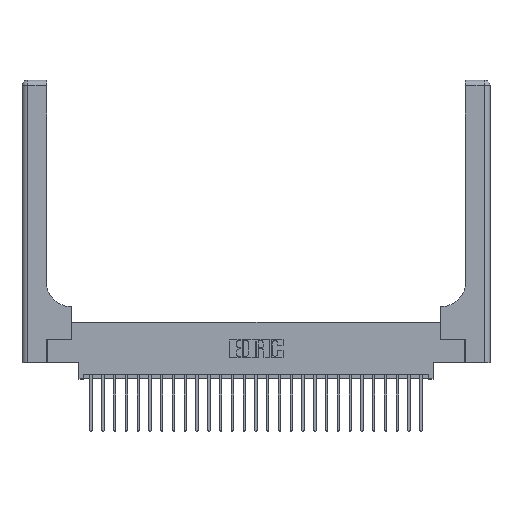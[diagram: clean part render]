
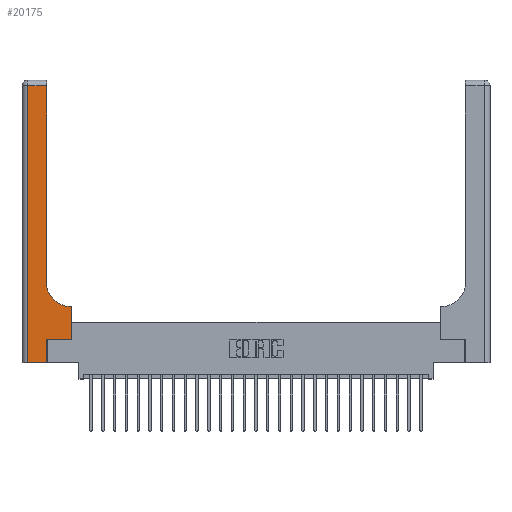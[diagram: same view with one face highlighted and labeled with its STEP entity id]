
A CAD part, top view. The second image highlights one B-rep face of the part: STEP entity #20175.
In plain terms, the highlighted planar face has unit normal (0, 0, 1).
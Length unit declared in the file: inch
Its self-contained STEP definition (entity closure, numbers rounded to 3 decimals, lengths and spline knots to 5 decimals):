
#98 = CARTESIAN_POINT ( 'NONE',  ( 0.528, 0.25, 0.37 ) ) ;
#495 = EDGE_CURVE ( 'NONE', #5238, #13865, #24114, .T. ) ;
#578 = VERTEX_POINT ( 'NONE', #21238 ) ;
#919 = ORIENTED_EDGE ( 'NONE', *, *, #9119, .T. ) ;
#1063 = CARTESIAN_POINT ( 'NONE',  ( 0.265, 0.25, 0.37 ) ) ;
#1071 = DIRECTION ( 'NONE',  ( 1., 0., 0. ) ) ;
#2001 = VERTEX_POINT ( 'NONE', #22235 ) ;
#2119 = VECTOR ( 'NONE', #13141, 39.37008 ) ;
#2160 = VECTOR ( 'NONE', #2380, 39.37008 ) ;
#2380 = DIRECTION ( 'NONE',  ( 0., -1., 0. ) ) ;
#2466 = VERTEX_POINT ( 'NONE', #25644 ) ;
#2586 = EDGE_CURVE ( 'NONE', #578, #5238, #10219, .T. ) ;
#4257 = CARTESIAN_POINT ( 'NONE',  ( 0.26, 2.94, 0.37 ) ) ;
#4840 = LINE ( 'NONE', #10431, #6106 ) ;
#4924 = CARTESIAN_POINT ( 'NONE',  ( 0.265, 0., 0.37 ) ) ;
#5238 = VERTEX_POINT ( 'NONE', #7798 ) ;
#5570 = ORIENTED_EDGE ( 'NONE', *, *, #13798, .T. ) ;
#5649 = ORIENTED_EDGE ( 'NONE', *, *, #495, .T. ) ;
#6106 = VECTOR ( 'NONE', #22444, 39.37008 ) ;
#6125 = ORIENTED_EDGE ( 'NONE', *, *, #25254, .T. ) ;
#7269 = EDGE_LOOP ( 'NONE', ( #13743, #919, #6125, #23512, #5649, #5570, #12803, #18125, #8104 ) ) ;
#7500 = LINE ( 'NONE', #17080, #2119 ) ;
#7531 = VERTEX_POINT ( 'NONE', #12950 ) ;
#7798 = CARTESIAN_POINT ( 'NONE',  ( 0.265, 0., 0.37 ) ) ;
#8031 = DIRECTION ( 'NONE',  ( 0., 0., -1. ) ) ;
#8104 = ORIENTED_EDGE ( 'NONE', *, *, #19860, .T. ) ;
#8174 = LINE ( 'NONE', #14430, #2160 ) ;
#8747 = CARTESIAN_POINT ( 'NONE',  ( 0., 2.94, 0.37 ) ) ;
#8979 = VERTEX_POINT ( 'NONE', #4257 ) ;
#9014 = CARTESIAN_POINT ( 'NONE',  ( 0.265, 0.25, 0.37 ) ) ;
#9119 = EDGE_CURVE ( 'NONE', #8979, #11363, #23045, .T. ) ;
#9296 = VECTOR ( 'NONE', #16214, 39.37008 ) ;
#10219 = LINE ( 'NONE', #13956, #14925 ) ;
#10431 = CARTESIAN_POINT ( 'NONE',  ( 0.26, 3., 0.37 ) ) ;
#10908 = AXIS2_PLACEMENT_3D ( 'NONE', #25143, #13137, #1071 ) ;
#10985 = DIRECTION ( 'NONE',  ( 0., 1., 0. ) ) ;
#11189 = VERTEX_POINT ( 'NONE', #16706 ) ;
#11363 = VERTEX_POINT ( 'NONE', #11869 ) ;
#11869 = CARTESIAN_POINT ( 'NONE',  ( 0.06, 2.94, 0.37 ) ) ;
#11971 = CARTESIAN_POINT ( 'NONE',  ( 0., 3., 0.37 ) ) ;
#12465 = EDGE_CURVE ( 'NONE', #7531, #2466, #7500, .T. ) ;
#12803 = ORIENTED_EDGE ( 'NONE', *, *, #21527, .T. ) ;
#12950 = CARTESIAN_POINT ( 'NONE',  ( 0.528, 0.6, 0.37 ) ) ;
#13097 = AXIS2_PLACEMENT_3D ( 'NONE', #11971, #8031, #22046 ) ;
#13137 = DIRECTION ( 'NONE',  ( 0., 0., -1. ) ) ;
#13141 = DIRECTION ( 'NONE',  ( -1., 0., 0. ) ) ;
#13294 = VECTOR ( 'NONE', #23034, 39.37008 ) ;
#13743 = ORIENTED_EDGE ( 'NONE', *, *, #22716, .T. ) ;
#13798 = EDGE_CURVE ( 'NONE', #13865, #2001, #17975, .T. ) ;
#13865 = VERTEX_POINT ( 'NONE', #1063 ) ;
#13956 = CARTESIAN_POINT ( 'NONE',  ( 0., 0., 0.37 ) ) ;
#14430 = CARTESIAN_POINT ( 'NONE',  ( 0.06, 3., 0.37 ) ) ;
#14925 = VECTOR ( 'NONE', #17988, 39.37008 ) ;
#15609 = FACE_OUTER_BOUND ( 'NONE', #7269, .T. ) ;
#16214 = DIRECTION ( 'NONE',  ( 0., 1., 0. ) ) ;
#16706 = CARTESIAN_POINT ( 'NONE',  ( 0.26, 0.85, 0.37 ) ) ;
#17080 = CARTESIAN_POINT ( 'NONE',  ( 0.26, 0.6, 0.37 ) ) ;
#17975 = LINE ( 'NONE', #9014, #13294 ) ;
#17988 = DIRECTION ( 'NONE',  ( 1., 0., 0. ) ) ;
#18125 = ORIENTED_EDGE ( 'NONE', *, *, #12465, .T. ) ;
#18340 = VECTOR ( 'NONE', #22765, 39.37008 ) ;
#19860 = EDGE_CURVE ( 'NONE', #2466, #11189, #22528, .T. ) ;
#20035 = PLANE ( 'NONE',  #13097 ) ;
#20175 = ADVANCED_FACE ( 'NONE', ( #15609 ), #20035, .F. ) ;
#21238 = CARTESIAN_POINT ( 'NONE',  ( 0.06, 0., 0.37 ) ) ;
#21527 = EDGE_CURVE ( 'NONE', #2001, #7531, #25932, .T. ) ;
#22046 = DIRECTION ( 'NONE',  ( -1., 0., 0. ) ) ;
#22235 = CARTESIAN_POINT ( 'NONE',  ( 0.528, 0.25, 0.37 ) ) ;
#22444 = DIRECTION ( 'NONE',  ( 0., 1., 0. ) ) ;
#22528 = CIRCLE ( 'NONE', #10908, 0.25 ) ;
#22716 = EDGE_CURVE ( 'NONE', #11189, #8979, #4840, .T. ) ;
#22765 = DIRECTION ( 'NONE',  ( -1., 0., 0. ) ) ;
#23034 = DIRECTION ( 'NONE',  ( 1., 0., 0. ) ) ;
#23045 = LINE ( 'NONE', #8747, #18340 ) ;
#23502 = VECTOR ( 'NONE', #10985, 39.37008 ) ;
#23512 = ORIENTED_EDGE ( 'NONE', *, *, #2586, .T. ) ;
#24114 = LINE ( 'NONE', #4924, #23502 ) ;
#25143 = CARTESIAN_POINT ( 'NONE',  ( 0.51, 0.85, 0.37 ) ) ;
#25254 = EDGE_CURVE ( 'NONE', #11363, #578, #8174, .T. ) ;
#25644 = CARTESIAN_POINT ( 'NONE',  ( 0.51, 0.6, 0.37 ) ) ;
#25932 = LINE ( 'NONE', #98, #9296 ) ;
